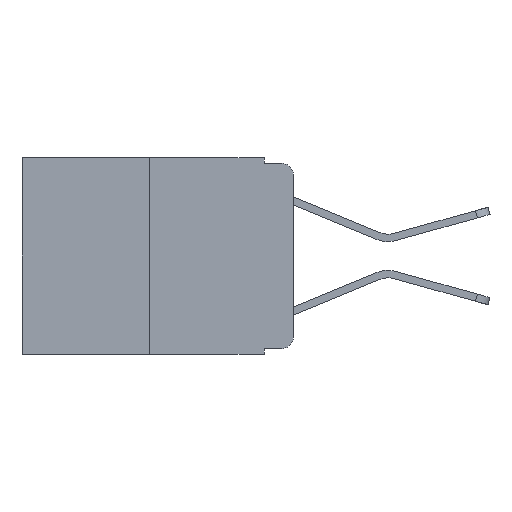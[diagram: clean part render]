
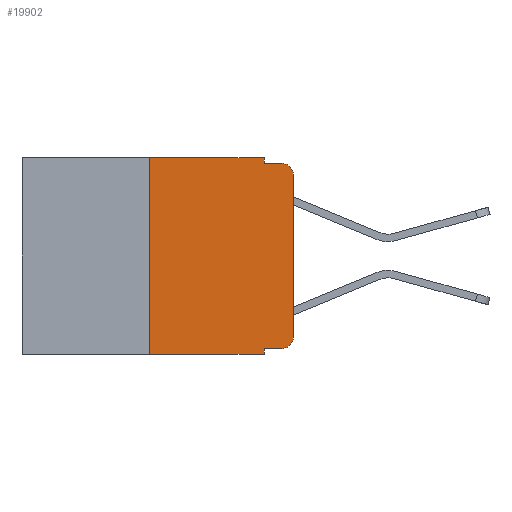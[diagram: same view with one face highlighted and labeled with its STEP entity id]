
A CAD part, left-side view. The second image highlights one B-rep face of the part: STEP entity #19902.
In plain terms, the highlighted planar face has unit normal (-1, 0, 0).
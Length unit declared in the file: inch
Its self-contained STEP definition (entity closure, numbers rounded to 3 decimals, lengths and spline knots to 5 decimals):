
#236 = CARTESIAN_POINT ( 'NONE',  ( 0., 0., 0. ) ) ;
#608 = VERTEX_POINT ( 'NONE', #20515 ) ;
#800 = DIRECTION ( 'NONE',  ( 0., -1., 0. ) ) ;
#808 = DIRECTION ( 'NONE',  ( -1., 0., 0. ) ) ;
#1223 = CARTESIAN_POINT ( 'NONE',  ( 0., 0.25, -0.343 ) ) ;
#1657 = CARTESIAN_POINT ( 'NONE',  ( 0., 0., -0.313 ) ) ;
#1697 = AXIS2_PLACEMENT_3D ( 'NONE', #3927, #5847, #18595 ) ;
#2007 = CARTESIAN_POINT ( 'NONE',  ( 0., 0.02, -0.333 ) ) ;
#2179 = LINE ( 'NONE', #22552, #7260 ) ;
#2556 = ORIENTED_EDGE ( 'NONE', *, *, #19030, .T. ) ;
#2584 = DIRECTION ( 'NONE',  ( 0., -1., 0. ) ) ;
#2929 = LINE ( 'NONE', #7438, #17615 ) ;
#3135 = EDGE_CURVE ( 'NONE', #12758, #608, #18759, .T. ) ;
#3839 = VECTOR ( 'NONE', #22197, 39.37008 ) ;
#3927 = CARTESIAN_POINT ( 'NONE',  ( 0., 0.473, 0. ) ) ;
#4169 = CARTESIAN_POINT ( 'NONE',  ( 0., 0.473, 0. ) ) ;
#4220 = VERTEX_POINT ( 'NONE', #8169 ) ;
#4528 = VECTOR ( 'NONE', #6091, 39.37008 ) ;
#4827 = EDGE_CURVE ( 'NONE', #17839, #9762, #11919, .T. ) ;
#5441 = DIRECTION ( 'NONE',  ( 0., -1., 0. ) ) ;
#5724 = LINE ( 'NONE', #19991, #23192 ) ;
#5742 = CARTESIAN_POINT ( 'NONE',  ( 0., 0.051, -0.01 ) ) ;
#5847 = DIRECTION ( 'NONE',  ( 1., 0., 0. ) ) ;
#6091 = DIRECTION ( 'NONE',  ( 0., -1., 0. ) ) ;
#6376 = FACE_OUTER_BOUND ( 'NONE', #7005, .T. ) ;
#6603 = CARTESIAN_POINT ( 'NONE',  ( 0., 0.051, 0. ) ) ;
#7005 = EDGE_LOOP ( 'NONE', ( #14661, #10468, #15790, #11559, #18091, #9048, #14384, #10218, #16087, #2556 ) ) ;
#7260 = VECTOR ( 'NONE', #2584, 39.37008 ) ;
#7438 = CARTESIAN_POINT ( 'NONE',  ( 0., 0.051, 0. ) ) ;
#7921 = DIRECTION ( 'NONE',  ( 0., 0., 1. ) ) ;
#8169 = CARTESIAN_POINT ( 'NONE',  ( 0., 0.051, -0.333 ) ) ;
#8780 = CARTESIAN_POINT ( 'NONE',  ( 0., 0., -0.03 ) ) ;
#9048 = ORIENTED_EDGE ( 'NONE', *, *, #12561, .F. ) ;
#9184 = LINE ( 'NONE', #22482, #18229 ) ;
#9629 = LINE ( 'NONE', #22777, #23279 ) ;
#9762 = VERTEX_POINT ( 'NONE', #5742 ) ;
#10218 = ORIENTED_EDGE ( 'NONE', *, *, #14156, .F. ) ;
#10468 = ORIENTED_EDGE ( 'NONE', *, *, #3135, .T. ) ;
#10592 = DIRECTION ( 'NONE',  ( -1., 0., 0. ) ) ;
#11107 = DIRECTION ( 'NONE',  ( 0., 0., -1. ) ) ;
#11467 = EDGE_CURVE ( 'NONE', #4220, #15273, #5724, .T. ) ;
#11559 = ORIENTED_EDGE ( 'NONE', *, *, #4827, .F. ) ;
#11763 = DIRECTION ( 'NONE',  ( 0., 0., 1. ) ) ;
#11769 = CARTESIAN_POINT ( 'NONE',  ( 0., 0.051, -0.343 ) ) ;
#11919 = LINE ( 'NONE', #20481, #3839 ) ;
#11985 = CARTESIAN_POINT ( 'NONE',  ( 0., 0.02, -0.03 ) ) ;
#12193 = VERTEX_POINT ( 'NONE', #14311 ) ;
#12561 = EDGE_CURVE ( 'NONE', #14613, #12193, #9184, .T. ) ;
#12758 = VERTEX_POINT ( 'NONE', #8780 ) ;
#13829 = DIRECTION ( 'NONE',  ( 0., 0., -1. ) ) ;
#14156 = EDGE_CURVE ( 'NONE', #4220, #17292, #2929, .T. ) ;
#14311 = CARTESIAN_POINT ( 'NONE',  ( 0., 0.25, 0. ) ) ;
#14384 = ORIENTED_EDGE ( 'NONE', *, *, #20090, .T. ) ;
#14394 = AXIS2_PLACEMENT_3D ( 'NONE', #21335, #10592, #23049 ) ;
#14613 = VERTEX_POINT ( 'NONE', #1223 ) ;
#14661 = ORIENTED_EDGE ( 'NONE', *, *, #21852, .T. ) ;
#14935 = PLANE ( 'NONE',  #1697 ) ;
#15273 = VERTEX_POINT ( 'NONE', #2007 ) ;
#15790 = ORIENTED_EDGE ( 'NONE', *, *, #18354, .F. ) ;
#16087 = ORIENTED_EDGE ( 'NONE', *, *, #11467, .T. ) ;
#16602 = VECTOR ( 'NONE', #7921, 39.37008 ) ;
#17092 = VERTEX_POINT ( 'NONE', #1657 ) ;
#17174 = LINE ( 'NONE', #236, #16602 ) ;
#17292 = VERTEX_POINT ( 'NONE', #11769 ) ;
#17615 = VECTOR ( 'NONE', #11107, 39.37008 ) ;
#17839 = VERTEX_POINT ( 'NONE', #6603 ) ;
#18091 = ORIENTED_EDGE ( 'NONE', *, *, #22763, .F. ) ;
#18229 = VECTOR ( 'NONE', #11763, 39.37008 ) ;
#18354 = EDGE_CURVE ( 'NONE', #9762, #608, #9629, .T. ) ;
#18595 = DIRECTION ( 'NONE',  ( 0., 0., -1. ) ) ;
#18759 = CIRCLE ( 'NONE', #22675, 0.02 ) ;
#19030 = EDGE_CURVE ( 'NONE', #15273, #17092, #19462, .T. ) ;
#19110 = LINE ( 'NONE', #4169, #4528 ) ;
#19462 = CIRCLE ( 'NONE', #14394, 0.02 ) ;
#19902 = ADVANCED_FACE ( 'NONE', ( #6376 ), #14935, .F. ) ;
#19991 = CARTESIAN_POINT ( 'NONE',  ( 0., 0.051, -0.333 ) ) ;
#20090 = EDGE_CURVE ( 'NONE', #14613, #17292, #2179, .T. ) ;
#20481 = CARTESIAN_POINT ( 'NONE',  ( 0., 0.051, 0. ) ) ;
#20515 = CARTESIAN_POINT ( 'NONE',  ( 0., 0.02, -0.01 ) ) ;
#21335 = CARTESIAN_POINT ( 'NONE',  ( 0., 0.02, -0.313 ) ) ;
#21852 = EDGE_CURVE ( 'NONE', #17092, #12758, #17174, .T. ) ;
#22197 = DIRECTION ( 'NONE',  ( 0., 0., -1. ) ) ;
#22482 = CARTESIAN_POINT ( 'NONE',  ( 0., 0.25, 0. ) ) ;
#22552 = CARTESIAN_POINT ( 'NONE',  ( 0., 0.473, -0.343 ) ) ;
#22675 = AXIS2_PLACEMENT_3D ( 'NONE', #11985, #808, #13829 ) ;
#22763 = EDGE_CURVE ( 'NONE', #12193, #17839, #19110, .T. ) ;
#22777 = CARTESIAN_POINT ( 'NONE',  ( 0., 0.051, -0.01 ) ) ;
#23049 = DIRECTION ( 'NONE',  ( 0., 0., -1. ) ) ;
#23192 = VECTOR ( 'NONE', #5441, 39.37008 ) ;
#23279 = VECTOR ( 'NONE', #800, 39.37008 ) ;
